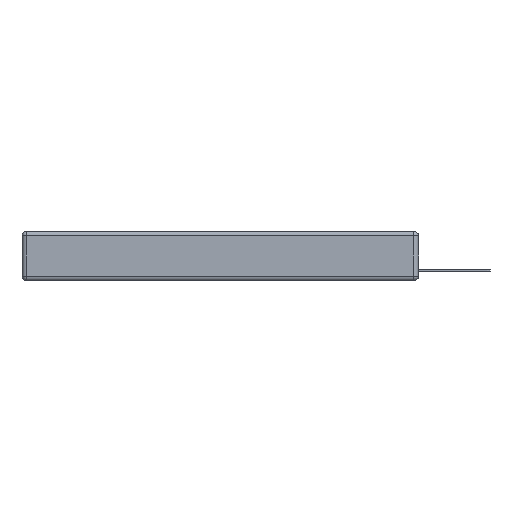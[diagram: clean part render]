
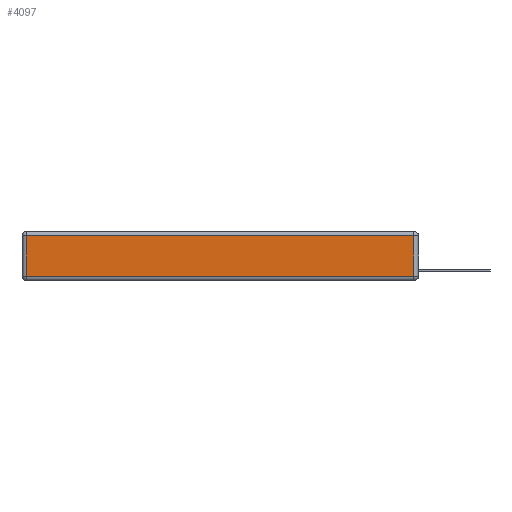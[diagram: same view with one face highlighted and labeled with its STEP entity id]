
A CAD part, left-side view. The second image highlights one B-rep face of the part: STEP entity #4097.
In plain terms, the highlighted planar face has unit normal (-1, 0, 0).
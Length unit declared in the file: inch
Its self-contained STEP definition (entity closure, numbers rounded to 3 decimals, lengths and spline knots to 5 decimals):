
#235 = CARTESIAN_POINT ( 'NONE',  ( 0., 0.03, -0.313 ) ) ;
#373 = DIRECTION ( 'NONE',  ( 0., 0., 1. ) ) ;
#484 = EDGE_CURVE ( 'NONE', #5704, #12552, #6641, .T. ) ;
#824 = CARTESIAN_POINT ( 'NONE',  ( 0., 2.72, -0.03 ) ) ;
#923 = AXIS2_PLACEMENT_3D ( 'NONE', #11174, #13450, #4554 ) ;
#1138 = VECTOR ( 'NONE', #373, 39.37008 ) ;
#2049 = LINE ( 'NONE', #2828, #11519 ) ;
#2304 = VECTOR ( 'NONE', #6623, 39.37008 ) ;
#2340 = CARTESIAN_POINT ( 'NONE',  ( 0., 0.03, -0.03 ) ) ;
#2566 = LINE ( 'NONE', #8325, #1138 ) ;
#2828 = CARTESIAN_POINT ( 'NONE',  ( 0., 0., -0.313 ) ) ;
#3082 = ORIENTED_EDGE ( 'NONE', *, *, #13514, .T. ) ;
#3278 = CARTESIAN_POINT ( 'NONE',  ( 0., 2.72, -0.313 ) ) ;
#4063 = DIRECTION ( 'NONE',  ( 0., 1., 0. ) ) ;
#4097 = ADVANCED_FACE ( 'NONE', ( #13585 ), #7871, .T. ) ;
#4554 = DIRECTION ( 'NONE',  ( 0., 0., 1. ) ) ;
#5124 = CARTESIAN_POINT ( 'NONE',  ( 0., 2.75, -0.03 ) ) ;
#5704 = VERTEX_POINT ( 'NONE', #824 ) ;
#6125 = DIRECTION ( 'NONE',  ( 0., -1., 0. ) ) ;
#6623 = DIRECTION ( 'NONE',  ( 0., 0., -1. ) ) ;
#6641 = LINE ( 'NONE', #11220, #2304 ) ;
#7871 = PLANE ( 'NONE',  #923 ) ;
#8306 = VECTOR ( 'NONE', #4063, 39.37008 ) ;
#8325 = CARTESIAN_POINT ( 'NONE',  ( 0., 0.03, -0.343 ) ) ;
#9544 = EDGE_CURVE ( 'NONE', #13279, #5704, #11995, .T. ) ;
#11174 = CARTESIAN_POINT ( 'NONE',  ( 0., 0., -0.343 ) ) ;
#11220 = CARTESIAN_POINT ( 'NONE',  ( 0., 2.72, -0.343 ) ) ;
#11519 = VECTOR ( 'NONE', #6125, 39.37008 ) ;
#11635 = ORIENTED_EDGE ( 'NONE', *, *, #14058, .T. ) ;
#11796 = ORIENTED_EDGE ( 'NONE', *, *, #9544, .T. ) ;
#11995 = LINE ( 'NONE', #5124, #8306 ) ;
#12552 = VERTEX_POINT ( 'NONE', #3278 ) ;
#12750 = EDGE_LOOP ( 'NONE', ( #3082, #11635, #11796, #14484 ) ) ;
#13279 = VERTEX_POINT ( 'NONE', #2340 ) ;
#13380 = VERTEX_POINT ( 'NONE', #235 ) ;
#13450 = DIRECTION ( 'NONE',  ( -1., 0., 0. ) ) ;
#13514 = EDGE_CURVE ( 'NONE', #12552, #13380, #2049, .T. ) ;
#13585 = FACE_OUTER_BOUND ( 'NONE', #12750, .T. ) ;
#14058 = EDGE_CURVE ( 'NONE', #13380, #13279, #2566, .T. ) ;
#14484 = ORIENTED_EDGE ( 'NONE', *, *, #484, .T. ) ;
